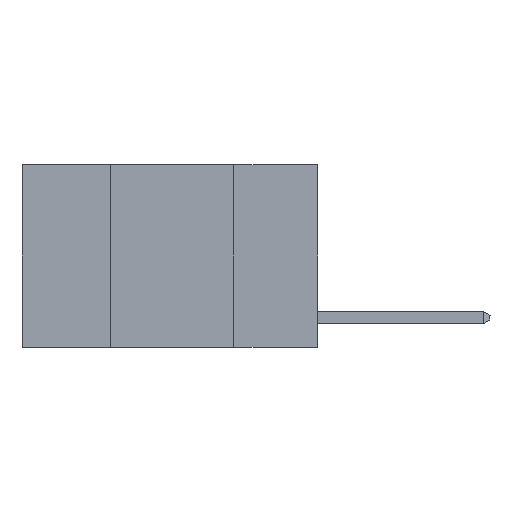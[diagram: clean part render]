
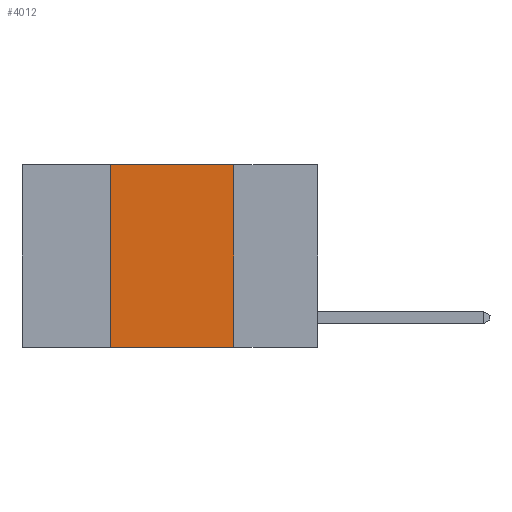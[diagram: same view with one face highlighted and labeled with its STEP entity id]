
A CAD part, left-side view. The second image highlights one B-rep face of the part: STEP entity #4012.
In plain terms, the highlighted planar face has unit normal (-1, 0, 0).
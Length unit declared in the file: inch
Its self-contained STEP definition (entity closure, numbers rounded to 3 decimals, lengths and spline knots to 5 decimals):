
#553 = DIRECTION ( 'NONE',  ( 1., 0., 0. ) ) ;
#688 = AXIS2_PLACEMENT_3D ( 'NONE', #6735, #553, #7752 ) ;
#716 = VECTOR ( 'NONE', #5395, 39.37008 ) ;
#750 = DIRECTION ( 'NONE',  ( 0., -1., 0. ) ) ;
#762 = LINE ( 'NONE', #3002, #11543 ) ;
#1616 = CARTESIAN_POINT ( 'NONE',  ( 0., 0.42, 0. ) ) ;
#1701 = LINE ( 'NONE', #2008, #716 ) ;
#1750 = EDGE_CURVE ( 'NONE', #8633, #6224, #1701, .T. ) ;
#2008 = CARTESIAN_POINT ( 'NONE',  ( 0., 0.6, 0. ) ) ;
#2249 = CARTESIAN_POINT ( 'NONE',  ( 0., 0.17, 0. ) ) ;
#3002 = CARTESIAN_POINT ( 'NONE',  ( 0., 0.42, 0. ) ) ;
#3062 = LINE ( 'NONE', #10725, #11107 ) ;
#4012 = ADVANCED_FACE ( 'NONE', ( #5177 ), #5714, .F. ) ;
#4032 = DIRECTION ( 'NONE',  ( 0., 0., 1. ) ) ;
#4162 = EDGE_CURVE ( 'NONE', #4809, #7299, #11587, .T. ) ;
#4809 = VERTEX_POINT ( 'NONE', #6803 ) ;
#5177 = FACE_OUTER_BOUND ( 'NONE', #10401, .T. ) ;
#5395 = DIRECTION ( 'NONE',  ( 0., -1., 0. ) ) ;
#5714 = PLANE ( 'NONE',  #688 ) ;
#5877 = CARTESIAN_POINT ( 'NONE',  ( 0., 0.17, -0.37 ) ) ;
#6224 = VERTEX_POINT ( 'NONE', #2249 ) ;
#6723 = ORIENTED_EDGE ( 'NONE', *, *, #11456, .F. ) ;
#6735 = CARTESIAN_POINT ( 'NONE',  ( 0., 0.6, 0. ) ) ;
#6803 = CARTESIAN_POINT ( 'NONE',  ( 0., 0.42, -0.37 ) ) ;
#7299 = VERTEX_POINT ( 'NONE', #5877 ) ;
#7526 = ORIENTED_EDGE ( 'NONE', *, *, #1750, .F. ) ;
#7717 = ORIENTED_EDGE ( 'NONE', *, *, #4162, .T. ) ;
#7752 = DIRECTION ( 'NONE',  ( 0., 0., -1. ) ) ;
#8633 = VERTEX_POINT ( 'NONE', #1616 ) ;
#8647 = VECTOR ( 'NONE', #750, 39.37008 ) ;
#10401 = EDGE_LOOP ( 'NONE', ( #6723, #7526, #10696, #7717 ) ) ;
#10696 = ORIENTED_EDGE ( 'NONE', *, *, #12632, .F. ) ;
#10725 = CARTESIAN_POINT ( 'NONE',  ( 0., 0.17, 0. ) ) ;
#11107 = VECTOR ( 'NONE', #11717, 39.37008 ) ;
#11456 = EDGE_CURVE ( 'NONE', #6224, #7299, #3062, .T. ) ;
#11543 = VECTOR ( 'NONE', #4032, 39.37008 ) ;
#11587 = LINE ( 'NONE', #11915, #8647 ) ;
#11717 = DIRECTION ( 'NONE',  ( 0., 0., -1. ) ) ;
#11915 = CARTESIAN_POINT ( 'NONE',  ( 0., 0.6, -0.37 ) ) ;
#12632 = EDGE_CURVE ( 'NONE', #4809, #8633, #762, .T. ) ;
